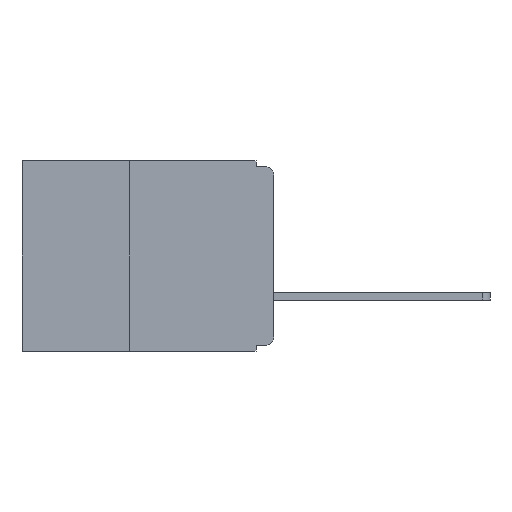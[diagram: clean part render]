
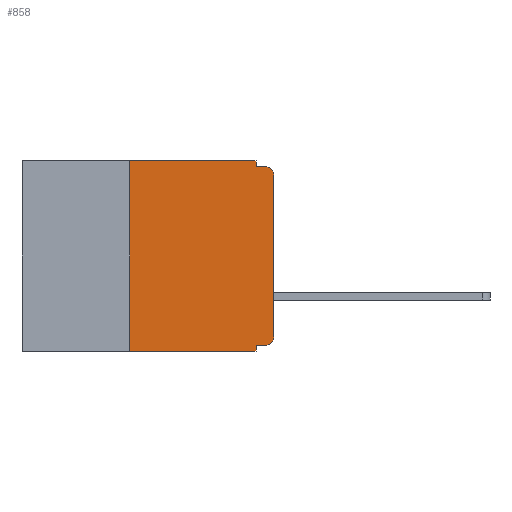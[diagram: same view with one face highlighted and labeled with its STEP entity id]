
A CAD part, left-side view. The second image highlights one B-rep face of the part: STEP entity #858.
In plain terms, the highlighted planar face has unit normal (-1, 0, 0).
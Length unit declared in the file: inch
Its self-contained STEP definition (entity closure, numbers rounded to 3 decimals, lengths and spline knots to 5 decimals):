
#478 = EDGE_CURVE ( 'NONE', #2510, #16847, #5388, .T. ) ;
#553 = DIRECTION ( 'NONE',  ( 0., 0., -1. ) ) ;
#611 = EDGE_CURVE ( 'NONE', #13207, #9621, #7346, .T. ) ;
#858 = ADVANCED_FACE ( 'NONE', ( #6256 ), #6357, .F. ) ;
#1178 = DIRECTION ( 'NONE',  ( -1., 0., 0. ) ) ;
#1452 = ORIENTED_EDGE ( 'NONE', *, *, #16939, .F. ) ;
#1860 = VERTEX_POINT ( 'NONE', #22478 ) ;
#1865 = VECTOR ( 'NONE', #15284, 39.37008 ) ;
#2510 = VERTEX_POINT ( 'NONE', #3763 ) ;
#2561 = ORIENTED_EDGE ( 'NONE', *, *, #17884, .F. ) ;
#3170 = CARTESIAN_POINT ( 'NONE',  ( 0., 0., -0.305 ) ) ;
#3763 = CARTESIAN_POINT ( 'NONE',  ( 0., 0.031, -0.32 ) ) ;
#4210 = EDGE_CURVE ( 'NONE', #8810, #1860, #12371, .T. ) ;
#4518 = ORIENTED_EDGE ( 'NONE', *, *, #8060, .T. ) ;
#4629 = CARTESIAN_POINT ( 'NONE',  ( 0., 0.25, -0.33 ) ) ;
#4746 = VECTOR ( 'NONE', #17448, 39.37008 ) ;
#4807 = EDGE_LOOP ( 'NONE', ( #4518, #9754, #1452, #11400, #20704, #2561, #7882, #17185, #22293, #8960 ) ) ;
#4821 = VECTOR ( 'NONE', #553, 39.37008 ) ;
#4892 = VERTEX_POINT ( 'NONE', #3170 ) ;
#5388 = LINE ( 'NONE', #5746, #4821 ) ;
#5477 = CARTESIAN_POINT ( 'NONE',  ( 0., 0.031, 0. ) ) ;
#5746 = CARTESIAN_POINT ( 'NONE',  ( 0., 0.031, -0.33 ) ) ;
#6008 = CIRCLE ( 'NONE', #8045, 0.015 ) ;
#6256 = FACE_OUTER_BOUND ( 'NONE', #4807, .T. ) ;
#6260 = VECTOR ( 'NONE', #16014, 39.37008 ) ;
#6311 = CARTESIAN_POINT ( 'NONE',  ( 0., 0., 0. ) ) ;
#6327 = AXIS2_PLACEMENT_3D ( 'NONE', #19796, #20682, #22139 ) ;
#6357 = PLANE ( 'NONE',  #6327 ) ;
#6777 = VECTOR ( 'NONE', #14181, 39.37008 ) ;
#7346 = LINE ( 'NONE', #12026, #6777 ) ;
#7753 = EDGE_CURVE ( 'NONE', #22211, #4892, #6008, .T. ) ;
#7882 = ORIENTED_EDGE ( 'NONE', *, *, #14534, .T. ) ;
#8045 = AXIS2_PLACEMENT_3D ( 'NONE', #9000, #21193, #10754 ) ;
#8060 = EDGE_CURVE ( 'NONE', #4892, #8810, #13387, .T. ) ;
#8227 = CARTESIAN_POINT ( 'NONE',  ( 0., 0., -0.32 ) ) ;
#8232 = CARTESIAN_POINT ( 'NONE',  ( 0., 0.015, -0.32 ) ) ;
#8393 = DIRECTION ( 'NONE',  ( 0., -1., 0. ) ) ;
#8810 = VERTEX_POINT ( 'NONE', #11845 ) ;
#8960 = ORIENTED_EDGE ( 'NONE', *, *, #7753, .T. ) ;
#9000 = CARTESIAN_POINT ( 'NONE',  ( 0., 0.015, -0.305 ) ) ;
#9026 = EDGE_CURVE ( 'NONE', #9621, #20999, #15604, .T. ) ;
#9605 = LINE ( 'NONE', #4629, #19498 ) ;
#9621 = VERTEX_POINT ( 'NONE', #18206 ) ;
#9754 = ORIENTED_EDGE ( 'NONE', *, *, #4210, .T. ) ;
#9877 = CARTESIAN_POINT ( 'NONE',  ( 0., 0.031, -0.01 ) ) ;
#10076 = CARTESIAN_POINT ( 'NONE',  ( 0., 0.031, -0.33 ) ) ;
#10387 = LINE ( 'NONE', #15318, #19175 ) ;
#10754 = DIRECTION ( 'NONE',  ( 0., 0., -1. ) ) ;
#11258 = LINE ( 'NONE', #8227, #1865 ) ;
#11400 = ORIENTED_EDGE ( 'NONE', *, *, #9026, .F. ) ;
#11760 = CARTESIAN_POINT ( 'NONE',  ( 0., 0.015, -0.025 ) ) ;
#11845 = CARTESIAN_POINT ( 'NONE',  ( 0., 0., -0.025 ) ) ;
#12026 = CARTESIAN_POINT ( 'NONE',  ( 0., 0.437, 0. ) ) ;
#12371 = CIRCLE ( 'NONE', #13255, 0.015 ) ;
#13207 = VERTEX_POINT ( 'NONE', #20155 ) ;
#13255 = AXIS2_PLACEMENT_3D ( 'NONE', #11760, #1178, #13525 ) ;
#13332 = EDGE_CURVE ( 'NONE', #22211, #2510, #11258, .T. ) ;
#13387 = LINE ( 'NONE', #6311, #17516 ) ;
#13406 = DIRECTION ( 'NONE',  ( 0., 0., 1. ) ) ;
#13525 = DIRECTION ( 'NONE',  ( 0., 0., -1. ) ) ;
#14181 = DIRECTION ( 'NONE',  ( 0., -1., 0. ) ) ;
#14534 = EDGE_CURVE ( 'NONE', #17374, #16847, #10387, .T. ) ;
#15080 = CARTESIAN_POINT ( 'NONE',  ( 0., 0.25, -0.33 ) ) ;
#15284 = DIRECTION ( 'NONE',  ( 0., 1., 0. ) ) ;
#15318 = CARTESIAN_POINT ( 'NONE',  ( 0., 0.437, -0.33 ) ) ;
#15604 = LINE ( 'NONE', #5477, #6260 ) ;
#16014 = DIRECTION ( 'NONE',  ( 0., 0., -1. ) ) ;
#16803 = DIRECTION ( 'NONE',  ( 0., 0., 1. ) ) ;
#16847 = VERTEX_POINT ( 'NONE', #10076 ) ;
#16939 = EDGE_CURVE ( 'NONE', #20999, #1860, #22232, .T. ) ;
#17185 = ORIENTED_EDGE ( 'NONE', *, *, #478, .F. ) ;
#17374 = VERTEX_POINT ( 'NONE', #15080 ) ;
#17448 = DIRECTION ( 'NONE',  ( 0., -1., 0. ) ) ;
#17516 = VECTOR ( 'NONE', #16803, 39.37008 ) ;
#17884 = EDGE_CURVE ( 'NONE', #17374, #13207, #9605, .T. ) ;
#18206 = CARTESIAN_POINT ( 'NONE',  ( 0., 0.031, 0. ) ) ;
#19175 = VECTOR ( 'NONE', #8393, 39.37008 ) ;
#19498 = VECTOR ( 'NONE', #13406, 39.37008 ) ;
#19796 = CARTESIAN_POINT ( 'NONE',  ( 0., 0.437, 0. ) ) ;
#20155 = CARTESIAN_POINT ( 'NONE',  ( 0., 0.25, 0. ) ) ;
#20682 = DIRECTION ( 'NONE',  ( 1., 0., 0. ) ) ;
#20704 = ORIENTED_EDGE ( 'NONE', *, *, #611, .F. ) ;
#20999 = VERTEX_POINT ( 'NONE', #9877 ) ;
#21193 = DIRECTION ( 'NONE',  ( -1., 0., 0. ) ) ;
#22139 = DIRECTION ( 'NONE',  ( 0., 0., -1. ) ) ;
#22211 = VERTEX_POINT ( 'NONE', #8232 ) ;
#22232 = LINE ( 'NONE', #22543, #4746 ) ;
#22293 = ORIENTED_EDGE ( 'NONE', *, *, #13332, .F. ) ;
#22478 = CARTESIAN_POINT ( 'NONE',  ( 0., 0.015, -0.01 ) ) ;
#22543 = CARTESIAN_POINT ( 'NONE',  ( 0., 0., -0.01 ) ) ;
